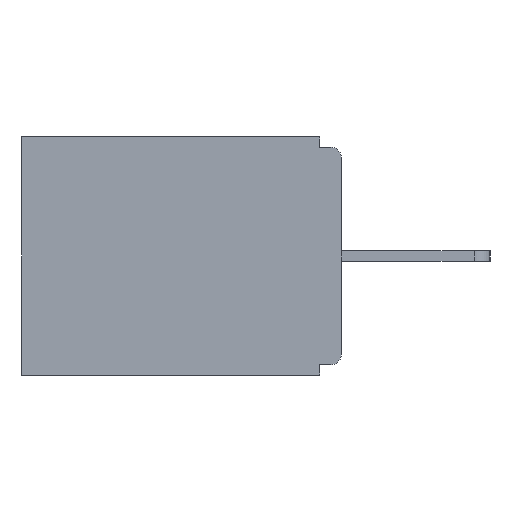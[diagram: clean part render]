
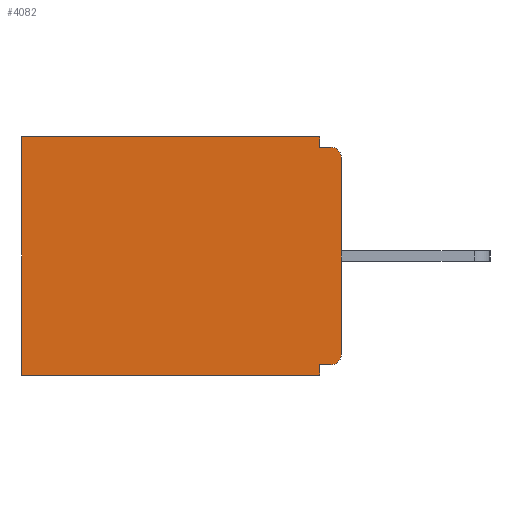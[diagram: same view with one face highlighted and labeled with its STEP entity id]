
A CAD part, left-side view. The second image highlights one B-rep face of the part: STEP entity #4082.
In plain terms, the highlighted planar face has unit normal (-1, 0, 0).
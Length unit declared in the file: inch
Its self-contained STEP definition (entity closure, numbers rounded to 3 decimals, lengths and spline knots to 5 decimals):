
#636 = EDGE_CURVE ( 'NONE', #7615, #5788, #2466, .T. ) ;
#668 = DIRECTION ( 'NONE',  ( 0., 1., 0. ) ) ;
#1686 = CARTESIAN_POINT ( 'NONE',  ( 0.298, 0.031, -0.343 ) ) ;
#2265 = EDGE_CURVE ( 'NONE', #9021, #3837, #2888, .T. ) ;
#2432 = AXIS2_PLACEMENT_3D ( 'NONE', #8168, #14828, #14726 ) ;
#2466 = LINE ( 'NONE', #15883, #4047 ) ;
#2549 = CARTESIAN_POINT ( 'NONE',  ( 0.298, 0.031, -0.343 ) ) ;
#2888 = LINE ( 'NONE', #3210, #11252 ) ;
#3210 = CARTESIAN_POINT ( 'NONE',  ( 0.298, 0., -0.328 ) ) ;
#3664 = VERTEX_POINT ( 'NONE', #14045 ) ;
#3837 = VERTEX_POINT ( 'NONE', #4527 ) ;
#3958 = DIRECTION ( 'NONE',  ( 0., 0., -1. ) ) ;
#4047 = VECTOR ( 'NONE', #668, 39.37008 ) ;
#4082 = ADVANCED_FACE ( 'NONE', ( #16711 ), #6198, .F. ) ;
#4527 = CARTESIAN_POINT ( 'NONE',  ( 0.298, 0.031, -0.328 ) ) ;
#4770 = VECTOR ( 'NONE', #3958, 39.37008 ) ;
#4869 = EDGE_CURVE ( 'NONE', #3664, #5788, #12365, .T. ) ;
#5481 = LINE ( 'NONE', #6685, #15032 ) ;
#5661 = CARTESIAN_POINT ( 'NONE',  ( 0.298, 0.015, -0.015 ) ) ;
#5788 = VERTEX_POINT ( 'NONE', #7667 ) ;
#5870 = LINE ( 'NONE', #6086, #15729 ) ;
#6086 = CARTESIAN_POINT ( 'NONE',  ( 0.298, 0., -0.015 ) ) ;
#6198 = PLANE ( 'NONE',  #2432 ) ;
#6638 = CARTESIAN_POINT ( 'NONE',  ( 0.298, 0.031, -0.343 ) ) ;
#6685 = CARTESIAN_POINT ( 'NONE',  ( 0.298, 0., 0. ) ) ;
#6736 = CARTESIAN_POINT ( 'NONE',  ( 0.298, 0., 0. ) ) ;
#6908 = DIRECTION ( 'NONE',  ( 0., 0., -1. ) ) ;
#7015 = ORIENTED_EDGE ( 'NONE', *, *, #18803, .F. ) ;
#7472 = ORIENTED_EDGE ( 'NONE', *, *, #19494, .F. ) ;
#7485 = ORIENTED_EDGE ( 'NONE', *, *, #4869, .T. ) ;
#7615 = VERTEX_POINT ( 'NONE', #1686 ) ;
#7667 = CARTESIAN_POINT ( 'NONE',  ( 0.298, 0.46, -0.343 ) ) ;
#7868 = DIRECTION ( 'NONE',  ( 0., 0., -1. ) ) ;
#8168 = CARTESIAN_POINT ( 'NONE',  ( 0.298, 0., 0. ) ) ;
#8516 = DIRECTION ( 'NONE',  ( 0., 1., 0. ) ) ;
#8606 = CARTESIAN_POINT ( 'NONE',  ( 0.298, 0.031, -0.015 ) ) ;
#8950 = CARTESIAN_POINT ( 'NONE',  ( 0.298, 0.031, 0. ) ) ;
#8995 = VECTOR ( 'NONE', #21319, 39.37008 ) ;
#9021 = VERTEX_POINT ( 'NONE', #10029 ) ;
#10029 = CARTESIAN_POINT ( 'NONE',  ( 0.298, 0.015, -0.328 ) ) ;
#10140 = VERTEX_POINT ( 'NONE', #5661 ) ;
#10552 = ORIENTED_EDGE ( 'NONE', *, *, #19177, .T. ) ;
#10603 = ORIENTED_EDGE ( 'NONE', *, *, #636, .F. ) ;
#10737 = CARTESIAN_POINT ( 'NONE',  ( 0.298, 0.015, -0.03 ) ) ;
#10789 = VECTOR ( 'NONE', #13390, 39.37008 ) ;
#10947 = CARTESIAN_POINT ( 'NONE',  ( 0.298, 0.46, 0. ) ) ;
#11252 = VECTOR ( 'NONE', #13278, 39.37008 ) ;
#12215 = EDGE_LOOP ( 'NONE', ( #10552, #7015, #12307, #14135, #7485, #10603, #16744, #21690, #13343, #7472 ) ) ;
#12307 = ORIENTED_EDGE ( 'NONE', *, *, #18443, .F. ) ;
#12325 = EDGE_CURVE ( 'NONE', #3837, #7615, #14509, .T. ) ;
#12365 = LINE ( 'NONE', #10947, #4770 ) ;
#12730 = CARTESIAN_POINT ( 'NONE',  ( 0.298, 0., -0.03 ) ) ;
#12842 = DIRECTION ( 'NONE',  ( 0., -1., 0. ) ) ;
#13278 = DIRECTION ( 'NONE',  ( 0., 1., 0. ) ) ;
#13343 = ORIENTED_EDGE ( 'NONE', *, *, #13483, .T. ) ;
#13390 = DIRECTION ( 'NONE',  ( 0., 0., -1. ) ) ;
#13483 = EDGE_CURVE ( 'NONE', #9021, #13808, #17371, .T. ) ;
#13808 = VERTEX_POINT ( 'NONE', #13934 ) ;
#13934 = CARTESIAN_POINT ( 'NONE',  ( 0.298, 0., -0.313 ) ) ;
#14045 = CARTESIAN_POINT ( 'NONE',  ( 0.298, 0.46, 0. ) ) ;
#14135 = ORIENTED_EDGE ( 'NONE', *, *, #21926, .T. ) ;
#14363 = DIRECTION ( 'NONE',  ( 0., 0., -1. ) ) ;
#14509 = LINE ( 'NONE', #2549, #8995 ) ;
#14726 = DIRECTION ( 'NONE',  ( 0., 0., -1. ) ) ;
#14828 = DIRECTION ( 'NONE',  ( 1., 0., 0. ) ) ;
#15032 = VECTOR ( 'NONE', #6908, 39.37008 ) ;
#15729 = VECTOR ( 'NONE', #12842, 39.37008 ) ;
#15883 = CARTESIAN_POINT ( 'NONE',  ( 0.298, 0., -0.343 ) ) ;
#16447 = AXIS2_PLACEMENT_3D ( 'NONE', #10737, #17700, #14363 ) ;
#16711 = FACE_OUTER_BOUND ( 'NONE', #12215, .T. ) ;
#16744 = ORIENTED_EDGE ( 'NONE', *, *, #12325, .F. ) ;
#17371 = CIRCLE ( 'NONE', #18430, 0.015 ) ;
#17700 = DIRECTION ( 'NONE',  ( -1., 0., 0. ) ) ;
#18430 = AXIS2_PLACEMENT_3D ( 'NONE', #19864, #21542, #7868 ) ;
#18443 = EDGE_CURVE ( 'NONE', #19102, #19064, #20097, .T. ) ;
#18575 = CIRCLE ( 'NONE', #16447, 0.015 ) ;
#18694 = VERTEX_POINT ( 'NONE', #12730 ) ;
#18803 = EDGE_CURVE ( 'NONE', #19064, #10140, #5870, .T. ) ;
#19064 = VERTEX_POINT ( 'NONE', #8606 ) ;
#19102 = VERTEX_POINT ( 'NONE', #8950 ) ;
#19177 = EDGE_CURVE ( 'NONE', #18694, #10140, #18575, .T. ) ;
#19494 = EDGE_CURVE ( 'NONE', #18694, #13808, #5481, .T. ) ;
#19864 = CARTESIAN_POINT ( 'NONE',  ( 0.298, 0.015, -0.313 ) ) ;
#20097 = LINE ( 'NONE', #6638, #10789 ) ;
#21319 = DIRECTION ( 'NONE',  ( 0., 0., -1. ) ) ;
#21542 = DIRECTION ( 'NONE',  ( -1., 0., 0. ) ) ;
#21560 = VECTOR ( 'NONE', #8516, 39.37008 ) ;
#21690 = ORIENTED_EDGE ( 'NONE', *, *, #2265, .F. ) ;
#21926 = EDGE_CURVE ( 'NONE', #19102, #3664, #21971, .T. ) ;
#21971 = LINE ( 'NONE', #6736, #21560 ) ;
